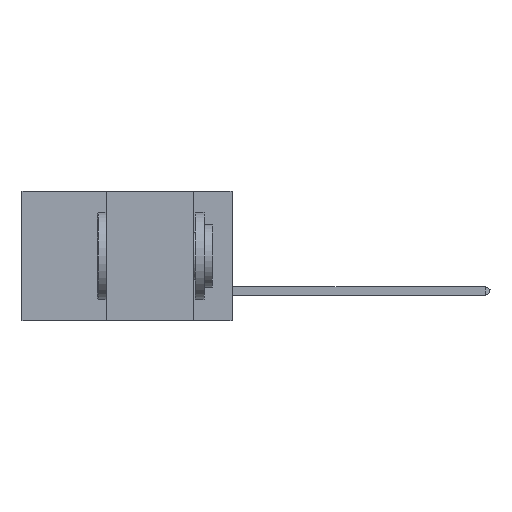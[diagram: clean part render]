
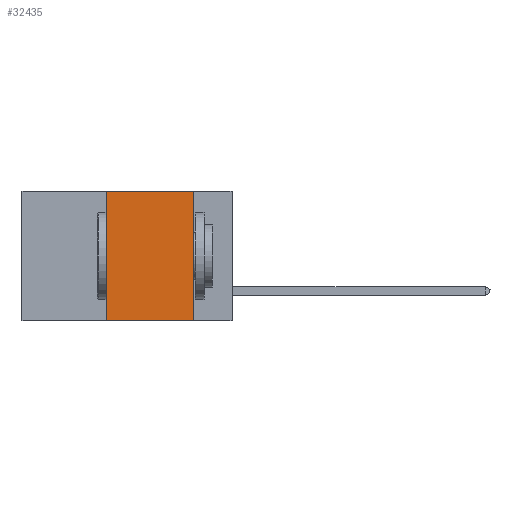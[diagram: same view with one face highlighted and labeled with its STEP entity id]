
A CAD part, left-side view. The second image highlights one B-rep face of the part: STEP entity #32435.
In plain terms, the highlighted planar face has unit normal (-1, 0, 0).
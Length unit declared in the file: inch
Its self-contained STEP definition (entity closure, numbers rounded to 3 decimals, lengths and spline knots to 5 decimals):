
#2459 = VECTOR ( 'NONE', #46361, 39.37008 ) ;
#3786 = CARTESIAN_POINT ( 'NONE',  ( 0., 0.6, 0. ) ) ;
#7408 = LINE ( 'NONE', #3786, #35294 ) ;
#7810 = DIRECTION ( 'NONE',  ( 0., -1., 0. ) ) ;
#8280 = ORIENTED_EDGE ( 'NONE', *, *, #27913, .F. ) ;
#9113 = DIRECTION ( 'NONE',  ( 0., 0., -1. ) ) ;
#11901 = FACE_OUTER_BOUND ( 'NONE', #48514, .T. ) ;
#12047 = PLANE ( 'NONE',  #49362 ) ;
#13125 = VERTEX_POINT ( 'NONE', #38258 ) ;
#15329 = VERTEX_POINT ( 'NONE', #25446 ) ;
#15810 = VERTEX_POINT ( 'NONE', #19166 ) ;
#16106 = CARTESIAN_POINT ( 'NONE',  ( 0., 0.6, -0.37 ) ) ;
#16934 = VECTOR ( 'NONE', #46669, 39.37008 ) ;
#18078 = ORIENTED_EDGE ( 'NONE', *, *, #45303, .T. ) ;
#19166 = CARTESIAN_POINT ( 'NONE',  ( 0., 0.11, 0. ) ) ;
#20143 = CARTESIAN_POINT ( 'NONE',  ( 0., 0.6, 0. ) ) ;
#20506 = DIRECTION ( 'NONE',  ( 0., 0., -1. ) ) ;
#23625 = LINE ( 'NONE', #26373, #2459 ) ;
#25446 = CARTESIAN_POINT ( 'NONE',  ( 0., 0.36, -0.37 ) ) ;
#26373 = CARTESIAN_POINT ( 'NONE',  ( 0., 0.36, 0. ) ) ;
#26789 = VECTOR ( 'NONE', #20506, 39.37008 ) ;
#27913 = EDGE_CURVE ( 'NONE', #15810, #13125, #45617, .T. ) ;
#30002 = EDGE_CURVE ( 'NONE', #49851, #15810, #7408, .T. ) ;
#30524 = CARTESIAN_POINT ( 'NONE',  ( 0., 0.36, 0. ) ) ;
#32435 = ADVANCED_FACE ( 'NONE', ( #11901 ), #12047, .F. ) ;
#34583 = ORIENTED_EDGE ( 'NONE', *, *, #45297, .F. ) ;
#35294 = VECTOR ( 'NONE', #7810, 39.37008 ) ;
#38258 = CARTESIAN_POINT ( 'NONE',  ( 0., 0.11, -0.37 ) ) ;
#39384 = ORIENTED_EDGE ( 'NONE', *, *, #30002, .F. ) ;
#39740 = CARTESIAN_POINT ( 'NONE',  ( 0., 0.11, 0. ) ) ;
#40550 = DIRECTION ( 'NONE',  ( 1., 0., 0. ) ) ;
#45297 = EDGE_CURVE ( 'NONE', #15329, #49851, #23625, .T. ) ;
#45303 = EDGE_CURVE ( 'NONE', #15329, #13125, #47858, .T. ) ;
#45617 = LINE ( 'NONE', #39740, #26789 ) ;
#46361 = DIRECTION ( 'NONE',  ( 0., 0., 1. ) ) ;
#46669 = DIRECTION ( 'NONE',  ( 0., -1., 0. ) ) ;
#47858 = LINE ( 'NONE', #16106, #16934 ) ;
#48514 = EDGE_LOOP ( 'NONE', ( #8280, #39384, #34583, #18078 ) ) ;
#49362 = AXIS2_PLACEMENT_3D ( 'NONE', #20143, #40550, #9113 ) ;
#49851 = VERTEX_POINT ( 'NONE', #30524 ) ;
